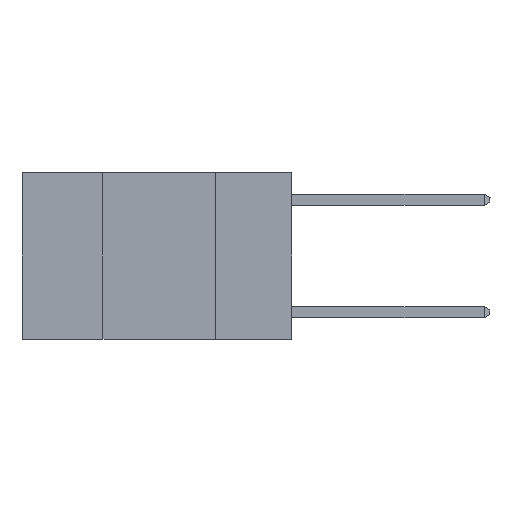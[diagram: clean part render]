
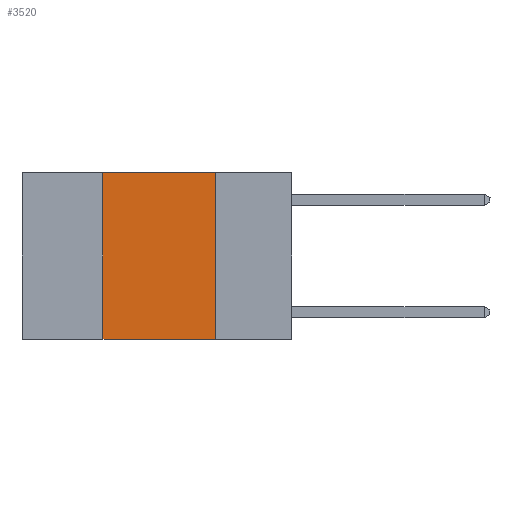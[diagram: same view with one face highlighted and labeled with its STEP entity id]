
A CAD part, left-side view. The second image highlights one B-rep face of the part: STEP entity #3520.
In plain terms, the highlighted planar face has unit normal (-1, 0, 0).
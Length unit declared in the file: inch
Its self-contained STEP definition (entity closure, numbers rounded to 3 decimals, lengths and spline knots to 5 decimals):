
#23 = VECTOR ( 'NONE', #10715, 39.37008 ) ;
#326 = ORIENTED_EDGE ( 'NONE', *, *, #7260, .T. ) ;
#566 = EDGE_LOOP ( 'NONE', ( #3318, #5256, #3690, #326 ) ) ;
#1404 = EDGE_CURVE ( 'NONE', #6564, #10375, #4433, .T. ) ;
#1638 = CARTESIAN_POINT ( 'NONE',  ( 0., 0.42, -0.37 ) ) ;
#1855 = CARTESIAN_POINT ( 'NONE',  ( 0., 0.6, 0. ) ) ;
#2157 = CARTESIAN_POINT ( 'NONE',  ( 0., 0.6, -0.37 ) ) ;
#2518 = CARTESIAN_POINT ( 'NONE',  ( 0., 0.17, 0. ) ) ;
#2873 = AXIS2_PLACEMENT_3D ( 'NONE', #7627, #9900, #11712 ) ;
#3207 = DIRECTION ( 'NONE',  ( 0., 0., 1. ) ) ;
#3318 = ORIENTED_EDGE ( 'NONE', *, *, #1404, .F. ) ;
#3387 = VECTOR ( 'NONE', #3808, 39.37008 ) ;
#3520 = ADVANCED_FACE ( 'NONE', ( #9829 ), #6635, .F. ) ;
#3690 = ORIENTED_EDGE ( 'NONE', *, *, #9402, .F. ) ;
#3808 = DIRECTION ( 'NONE',  ( 0., -1., 0. ) ) ;
#4066 = CARTESIAN_POINT ( 'NONE',  ( 0., 0.42, 0. ) ) ;
#4211 = CARTESIAN_POINT ( 'NONE',  ( 0., 0.17, -0.37 ) ) ;
#4433 = LINE ( 'NONE', #2518, #23 ) ;
#5256 = ORIENTED_EDGE ( 'NONE', *, *, #7494, .F. ) ;
#5890 = VERTEX_POINT ( 'NONE', #12343 ) ;
#5943 = CARTESIAN_POINT ( 'NONE',  ( 0., 0.17, 0. ) ) ;
#6360 = DIRECTION ( 'NONE',  ( 0., -1., 0. ) ) ;
#6564 = VERTEX_POINT ( 'NONE', #5943 ) ;
#6635 = PLANE ( 'NONE',  #2873 ) ;
#7260 = EDGE_CURVE ( 'NONE', #9648, #10375, #8415, .T. ) ;
#7494 = EDGE_CURVE ( 'NONE', #5890, #6564, #12941, .T. ) ;
#7621 = VECTOR ( 'NONE', #6360, 39.37008 ) ;
#7627 = CARTESIAN_POINT ( 'NONE',  ( 0., 0.6, 0. ) ) ;
#8415 = LINE ( 'NONE', #2157, #7621 ) ;
#9402 = EDGE_CURVE ( 'NONE', #9648, #5890, #12262, .T. ) ;
#9648 = VERTEX_POINT ( 'NONE', #1638 ) ;
#9829 = FACE_OUTER_BOUND ( 'NONE', #566, .T. ) ;
#9900 = DIRECTION ( 'NONE',  ( 1., 0., 0. ) ) ;
#10375 = VERTEX_POINT ( 'NONE', #4211 ) ;
#10715 = DIRECTION ( 'NONE',  ( 0., 0., -1. ) ) ;
#10935 = VECTOR ( 'NONE', #3207, 39.37008 ) ;
#11712 = DIRECTION ( 'NONE',  ( 0., 0., -1. ) ) ;
#12262 = LINE ( 'NONE', #4066, #10935 ) ;
#12343 = CARTESIAN_POINT ( 'NONE',  ( 0., 0.42, 0. ) ) ;
#12941 = LINE ( 'NONE', #1855, #3387 ) ;
